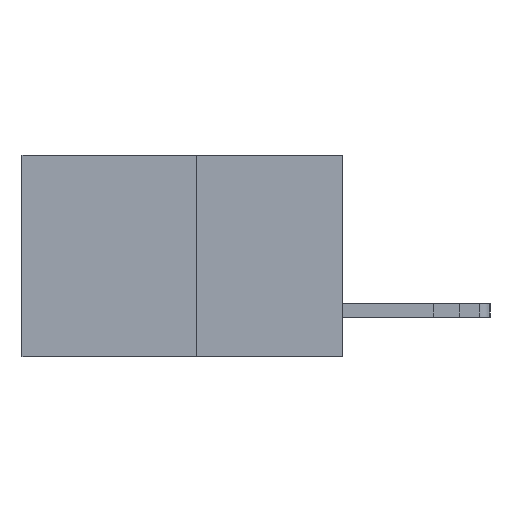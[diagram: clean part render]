
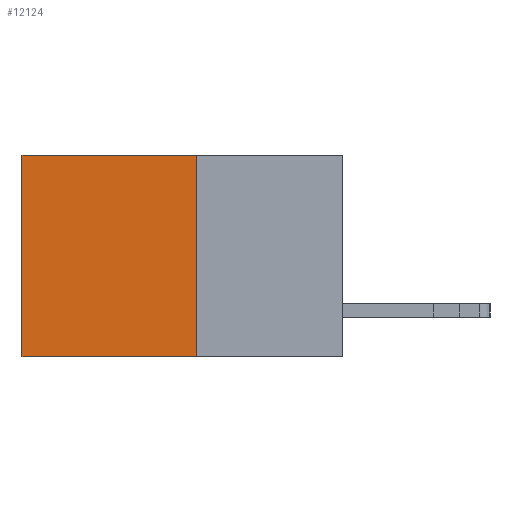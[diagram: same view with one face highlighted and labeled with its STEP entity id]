
A CAD part, left-side view. The second image highlights one B-rep face of the part: STEP entity #12124.
In plain terms, the highlighted planar face has unit normal (-1, 0, 0).
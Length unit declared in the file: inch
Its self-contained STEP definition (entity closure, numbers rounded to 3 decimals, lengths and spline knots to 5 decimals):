
#357 = ORIENTED_EDGE ( 'NONE', *, *, #16922, .T. ) ;
#724 = LINE ( 'NONE', #17806, #16537 ) ;
#1921 = CARTESIAN_POINT ( 'NONE',  ( 0.277, 0.27, -0.37 ) ) ;
#4448 = PLANE ( 'NONE',  #13180 ) ;
#5163 = VERTEX_POINT ( 'NONE', #11246 ) ;
#6018 = DIRECTION ( 'NONE',  ( 0., 0., -1. ) ) ;
#6740 = EDGE_LOOP ( 'NONE', ( #7399, #10126, #12589, #357 ) ) ;
#7399 = ORIENTED_EDGE ( 'NONE', *, *, #13387, .T. ) ;
#7693 = VECTOR ( 'NONE', #11068, 39.37008 ) ;
#8016 = FACE_OUTER_BOUND ( 'NONE', #6740, .T. ) ;
#8239 = DIRECTION ( 'NONE',  ( 0., 0., -1. ) ) ;
#8681 = DIRECTION ( 'NONE',  ( 0., 0., -1. ) ) ;
#8962 = CARTESIAN_POINT ( 'NONE',  ( 0.277, 0.27, -0.37 ) ) ;
#9387 = CARTESIAN_POINT ( 'NONE',  ( 0.277, 0.59, -0.37 ) ) ;
#10126 = ORIENTED_EDGE ( 'NONE', *, *, #16547, .F. ) ;
#11068 = DIRECTION ( 'NONE',  ( 0., 1., 0. ) ) ;
#11246 = CARTESIAN_POINT ( 'NONE',  ( 0.277, 0.27, -0.37 ) ) ;
#12124 = ADVANCED_FACE ( 'NONE', ( #8016 ), #4448, .F. ) ;
#12189 = LINE ( 'NONE', #1921, #7693 ) ;
#12458 = VECTOR ( 'NONE', #8239, 39.37008 ) ;
#12573 = VERTEX_POINT ( 'NONE', #9387 ) ;
#12589 = ORIENTED_EDGE ( 'NONE', *, *, #12968, .F. ) ;
#12643 = LINE ( 'NONE', #14997, #16216 ) ;
#12734 = CARTESIAN_POINT ( 'NONE',  ( 0.277, 0.59, -0.37 ) ) ;
#12921 = LINE ( 'NONE', #12734, #12458 ) ;
#12968 = EDGE_CURVE ( 'NONE', #13702, #5163, #724, .T. ) ;
#13180 = AXIS2_PLACEMENT_3D ( 'NONE', #8962, #15103, #6018 ) ;
#13387 = EDGE_CURVE ( 'NONE', #13503, #12573, #12921, .T. ) ;
#13503 = VERTEX_POINT ( 'NONE', #14623 ) ;
#13702 = VERTEX_POINT ( 'NONE', #16532 ) ;
#14623 = CARTESIAN_POINT ( 'NONE',  ( 0.277, 0.59, 0. ) ) ;
#14997 = CARTESIAN_POINT ( 'NONE',  ( 0.277, 0.27, 0. ) ) ;
#15103 = DIRECTION ( 'NONE',  ( 1., 0., 0. ) ) ;
#16216 = VECTOR ( 'NONE', #19556, 39.37008 ) ;
#16532 = CARTESIAN_POINT ( 'NONE',  ( 0.277, 0.27, 0. ) ) ;
#16537 = VECTOR ( 'NONE', #8681, 39.37008 ) ;
#16547 = EDGE_CURVE ( 'NONE', #5163, #12573, #12189, .T. ) ;
#16922 = EDGE_CURVE ( 'NONE', #13702, #13503, #12643, .T. ) ;
#17806 = CARTESIAN_POINT ( 'NONE',  ( 0.277, 0.27, -0.37 ) ) ;
#19556 = DIRECTION ( 'NONE',  ( 0., 1., 0. ) ) ;
